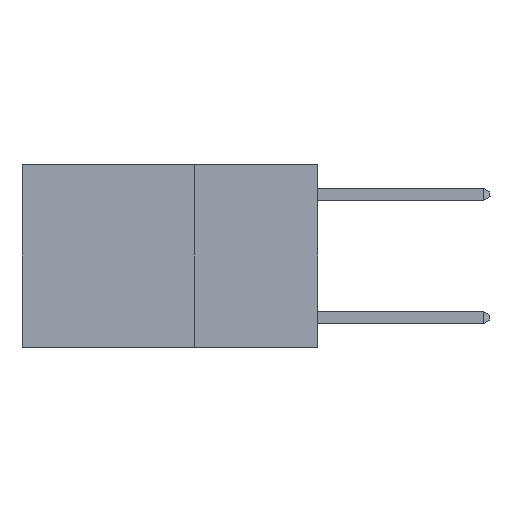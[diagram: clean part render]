
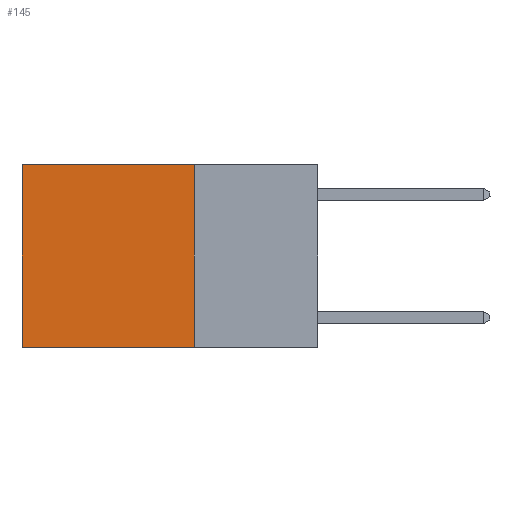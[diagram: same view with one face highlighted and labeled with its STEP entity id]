
A CAD part, left-side view. The second image highlights one B-rep face of the part: STEP entity #145.
In plain terms, the highlighted planar face has unit normal (-1, 0, 0).
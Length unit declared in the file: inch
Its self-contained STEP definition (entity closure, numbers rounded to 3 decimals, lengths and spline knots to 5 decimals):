
#21 = ORIENTED_EDGE ( 'NONE', *, *, #3230, .F. ) ;
#42 = ORIENTED_EDGE ( 'NONE', *, *, #1897, .T. ) ;
#51 = ORIENTED_EDGE ( 'NONE', *, *, #7283, .F. ) ;
#145 = ADVANCED_FACE ( 'NONE', ( #3481 ), #3045, .F. ) ;
#320 = ORIENTED_EDGE ( 'NONE', *, *, #5858, .T. ) ;
#409 = CARTESIAN_POINT ( 'NONE',  ( 0.2625, 0.25, 0. ) ) ;
#624 = VECTOR ( 'NONE', #1473, 39.37008 ) ;
#1065 = VERTEX_POINT ( 'NONE', #5769 ) ;
#1473 = DIRECTION ( 'NONE',  ( 0., 1., 0. ) ) ;
#1561 = EDGE_LOOP ( 'NONE', ( #320, #21, #51, #42 ) ) ;
#1897 = EDGE_CURVE ( 'NONE', #7334, #8468, #2739, .T. ) ;
#2739 = LINE ( 'NONE', #5200, #6401 ) ;
#2938 = CARTESIAN_POINT ( 'NONE',  ( 0.2625, 0.6, -0.37 ) ) ;
#3045 = PLANE ( 'NONE',  #7588 ) ;
#3121 = CARTESIAN_POINT ( 'NONE',  ( 0.2625, 0.25, 0. ) ) ;
#3230 = EDGE_CURVE ( 'NONE', #1065, #3827, #8601, .T. ) ;
#3457 = VECTOR ( 'NONE', #8530, 39.37008 ) ;
#3481 = FACE_OUTER_BOUND ( 'NONE', #1561, .T. ) ;
#3827 = VERTEX_POINT ( 'NONE', #2938 ) ;
#3858 = DIRECTION ( 'NONE',  ( 0., 0., -1. ) ) ;
#3960 = DIRECTION ( 'NONE',  ( 1., 0., 0. ) ) ;
#4298 = DIRECTION ( 'NONE',  ( 0., 0., -1. ) ) ;
#4614 = LINE ( 'NONE', #9207, #6434 ) ;
#4761 = CARTESIAN_POINT ( 'NONE',  ( 0.2625, 0.25, 0. ) ) ;
#5200 = CARTESIAN_POINT ( 'NONE',  ( 0.2625, 0.25, 0. ) ) ;
#5769 = CARTESIAN_POINT ( 'NONE',  ( 0.2625, 0.25, -0.37 ) ) ;
#5858 = EDGE_CURVE ( 'NONE', #8468, #3827, #4614, .T. ) ;
#6165 = CARTESIAN_POINT ( 'NONE',  ( 0.2625, 0.25, -0.37 ) ) ;
#6401 = VECTOR ( 'NONE', #9745, 39.37008 ) ;
#6434 = VECTOR ( 'NONE', #3858, 39.37008 ) ;
#7024 = CARTESIAN_POINT ( 'NONE',  ( 0.2625, 0.6, 0. ) ) ;
#7283 = EDGE_CURVE ( 'NONE', #7334, #1065, #7314, .T. ) ;
#7314 = LINE ( 'NONE', #3121, #3457 ) ;
#7334 = VERTEX_POINT ( 'NONE', #4761 ) ;
#7588 = AXIS2_PLACEMENT_3D ( 'NONE', #409, #3960, #4298 ) ;
#8468 = VERTEX_POINT ( 'NONE', #7024 ) ;
#8530 = DIRECTION ( 'NONE',  ( 0., 0., -1. ) ) ;
#8601 = LINE ( 'NONE', #6165, #624 ) ;
#9207 = CARTESIAN_POINT ( 'NONE',  ( 0.2625, 0.6, 0. ) ) ;
#9745 = DIRECTION ( 'NONE',  ( 0., 1., 0. ) ) ;
